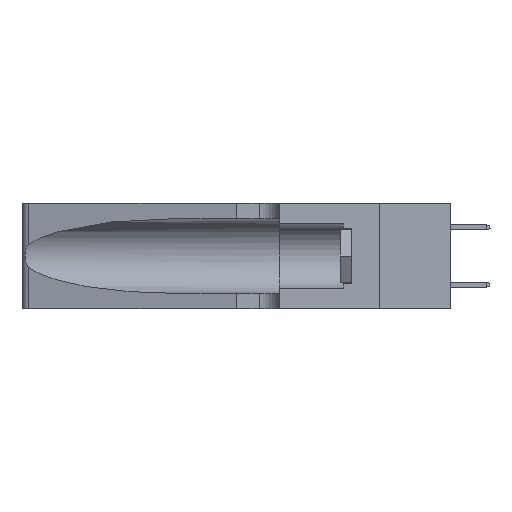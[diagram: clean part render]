
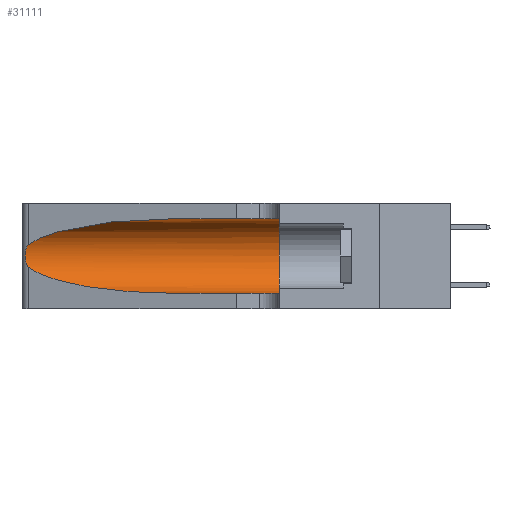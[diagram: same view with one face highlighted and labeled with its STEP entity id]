
A CAD part, left-side view. The second image highlights one B-rep face of the part: STEP entity #31111.
In plain terms, the highlighted cylindrical face has radius 3.308 mm (diameter 6.617 mm), a partial arc.
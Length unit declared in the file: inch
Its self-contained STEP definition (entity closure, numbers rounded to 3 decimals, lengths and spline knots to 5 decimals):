
#854 = CARTESIAN_POINT ( 'NONE',  ( 0.1305, 0.35, 0.185 ) ) ;
#1139 = CARTESIAN_POINT ( 'NONE',  ( 0.26075, 1.23896, 0.19203 ) ) ;
#1868 = VERTEX_POINT ( 'NONE', #34511 ) ;
#2355 = LINE ( 'NONE', #13602, #23605 ) ;
#2614 = EDGE_CURVE ( 'NONE', #1868, #17854, #2355, .T. ) ;
#2832 = CARTESIAN_POINT ( 'NONE',  ( 0.2373, 1.15595, 0.08982 ) ) ;
#3173 = EDGE_CURVE ( 'NONE', #36291, #3364, #33164, .T. ) ;
#3364 = VERTEX_POINT ( 'NONE', #32376 ) ;
#3614 = DIRECTION ( 'NONE',  ( 0., -1., 0. ) ) ;
#3705 = CARTESIAN_POINT ( 'NONE',  ( 0.25487, 1.22718, 0.14631 ) ) ;
#4072 = CARTESIAN_POINT ( 'NONE',  ( 0.25789, 1.23486, 0.15765 ) ) ;
#4599 = AXIS2_PLACEMENT_3D ( 'NONE', #854, #31383, #23393 ) ;
#6283 = CARTESIAN_POINT ( 'NONE',  ( 0.26018, 1.23835, 0.19895 ) ) ;
#7007 = CARTESIAN_POINT ( 'NONE',  ( 0.25856, 1.23593, 0.16098 ) ) ;
#7128 = EDGE_CURVE ( 'NONE', #21817, #22621, #12790, .T. ) ;
#7644 = CARTESIAN_POINT ( 'NONE',  ( 0.1305, 0.72297, 0.31525 ) ) ;
#8436 = EDGE_CURVE ( 'NONE', #22621, #1868, #34440, .T. ) ;
#10392 = CARTESIAN_POINT ( 'NONE',  ( 0.25487, 1.22718, 0.22369 ) ) ;
#10560 = DIRECTION ( 'NONE',  ( 0., -1., 0. ) ) ;
#11027 = EDGE_LOOP ( 'NONE', ( #31262, #28296, #20277, #20104, #32506, #25025 ) ) ;
#12395 = CARTESIAN_POINT ( 'NONE',  ( 0.26075, 1.23896, 0.178 ) ) ;
#12790 = B_SPLINE_CURVE_WITH_KNOTS ( 'NONE', 3,
 ( #23844, #32386, #25916, #26450, #17770, #6283, #1139, #12395, #29060, #7007, #4072, #34982, #23128, #3705 ),
 .UNSPECIFIED., .F., .F.,
 ( 4, 2, 2, 2, 2, 2, 4 ),
 ( 0., 0.00027, 0.00053, 0.00107, 0.0016, 0.00187, 0.00214 ),
 .UNSPECIFIED. ) ;
#13181 = CARTESIAN_POINT ( 'NONE',  ( 0.1305, 0.72297, 0.31525 ) ) ;
#13383 = DIRECTION ( 'NONE',  ( 0., 0., -1. ) ) ;
#13602 = CARTESIAN_POINT ( 'NONE',  ( 0.1305, 1.61858, 0.05475 ) ) ;
#14117 = CARTESIAN_POINT ( 'NONE',  ( 0.1305, 1.61858, 0.185 ) ) ;
#15745 = EDGE_CURVE ( 'NONE', #3364, #17854, #17589, .T. ) ;
#16351 = CYLINDRICAL_SURFACE ( 'NONE', #26923, 0.13025 ) ;
#16518 = CARTESIAN_POINT ( 'NONE',  ( 0.1305, 0.72297, 0.05475 ) ) ;
#17589 = CIRCLE ( 'NONE', #4599, 0.13025 ) ;
#17770 = CARTESIAN_POINT ( 'NONE',  ( 0.25854, 1.2359, 0.20912 ) ) ;
#17854 = VERTEX_POINT ( 'NONE', #24832 ) ;
#19271 = CARTESIAN_POINT ( 'NONE',  ( 0.25487, 1.22718, 0.14631 ) ) ;
#20104 = ORIENTED_EDGE ( 'NONE', *, *, #2614, .T. ) ;
#20277 = ORIENTED_EDGE ( 'NONE', *, *, #8436, .T. ) ;
#21718 = DIRECTION ( 'NONE',  ( 0., -1., 0. ) ) ;
#21817 = VERTEX_POINT ( 'NONE', #34972 ) ;
#22012 = CARTESIAN_POINT ( 'NONE',  ( 0.1305, 1.61858, 0.31525 ) ) ;
#22158 = VECTOR ( 'NONE', #10560, 39.37008 ) ;
#22621 = VERTEX_POINT ( 'NONE', #32098 ) ;
#23128 = CARTESIAN_POINT ( 'NONE',  ( 0.25555, 1.22993, 0.14849 ) ) ;
#23393 = DIRECTION ( 'NONE',  ( 0., 0., 1. ) ) ;
#23605 = VECTOR ( 'NONE', #3614, 39.37008 ) ;
#23844 = CARTESIAN_POINT ( 'NONE',  ( 0.25487, 1.22718, 0.22369 ) ) ;
#24463 = CARTESIAN_POINT ( 'NONE',  ( 0.18966, 0.96281, 0.31525 ) ) ;
#24832 = CARTESIAN_POINT ( 'NONE',  ( 0.1305, 0.35, 0.05475 ) ) ;
#24843 = CARTESIAN_POINT ( 'NONE',  ( 0.2373, 1.15595, 0.28018 ) ) ;
#24992 = EDGE_CURVE ( 'NONE', #36291, #21817, #26639, .T. ) ;
#25025 = ORIENTED_EDGE ( 'NONE', *, *, #3173, .F. ) ;
#25916 = CARTESIAN_POINT ( 'NONE',  ( 0.25639, 1.23184, 0.21858 ) ) ;
#26450 = CARTESIAN_POINT ( 'NONE',  ( 0.25787, 1.23484, 0.2124 ) ) ;
#26639 =( BOUNDED_CURVE ( )  B_SPLINE_CURVE ( 3, ( #13181, #24463, #24843, #10392 ),
 .UNSPECIFIED., .F., .F. ) 
 B_SPLINE_CURVE_WITH_KNOTS ( ( 4, 4 ),
 ( 1.5708, 2.84003 ),
 .UNSPECIFIED. ) 
 CURVE ( )  GEOMETRIC_REPRESENTATION_ITEM ( )  RATIONAL_B_SPLINE_CURVE ( ( 1., 0.87, 0.87, 1. ) ) 
 REPRESENTATION_ITEM ( '' )  );
#26923 = AXIS2_PLACEMENT_3D ( 'NONE', #14117, #21718, #13383 ) ;
#28162 = CARTESIAN_POINT ( 'NONE',  ( 0.18966, 0.96281, 0.05475 ) ) ;
#28191 = FACE_OUTER_BOUND ( 'NONE', #11027, .T. ) ;
#28296 = ORIENTED_EDGE ( 'NONE', *, *, #7128, .T. ) ;
#29060 = CARTESIAN_POINT ( 'NONE',  ( 0.26017, 1.23833, 0.17102 ) ) ;
#31111 = ADVANCED_FACE ( 'NONE', ( #28191 ), #16351, .F. ) ;
#31262 = ORIENTED_EDGE ( 'NONE', *, *, #24992, .T. ) ;
#31383 = DIRECTION ( 'NONE',  ( 0., 1., 0. ) ) ;
#32098 = CARTESIAN_POINT ( 'NONE',  ( 0.25487, 1.22718, 0.14631 ) ) ;
#32376 = CARTESIAN_POINT ( 'NONE',  ( 0.1305, 0.35, 0.31525 ) ) ;
#32386 = CARTESIAN_POINT ( 'NONE',  ( 0.25555, 1.22994, 0.2215 ) ) ;
#32506 = ORIENTED_EDGE ( 'NONE', *, *, #15745, .F. ) ;
#33164 = LINE ( 'NONE', #22012, #22158 ) ;
#34440 =( BOUNDED_CURVE ( )  B_SPLINE_CURVE ( 3, ( #19271, #2832, #28162, #16518 ),
 .UNSPECIFIED., .F., .T. ) 
 B_SPLINE_CURVE_WITH_KNOTS ( ( 4, 4 ),
 ( 3.44316, 4.71239 ),
 .UNSPECIFIED. ) 
 CURVE ( )  GEOMETRIC_REPRESENTATION_ITEM ( )  RATIONAL_B_SPLINE_CURVE ( ( 1., 0.87, 0.87, 1. ) ) 
 REPRESENTATION_ITEM ( '' )  );
#34511 = CARTESIAN_POINT ( 'NONE',  ( 0.1305, 0.72297, 0.05475 ) ) ;
#34972 = CARTESIAN_POINT ( 'NONE',  ( 0.25487, 1.22718, 0.22369 ) ) ;
#34982 = CARTESIAN_POINT ( 'NONE',  ( 0.25639, 1.23186, 0.15144 ) ) ;
#36291 = VERTEX_POINT ( 'NONE', #7644 ) ;
